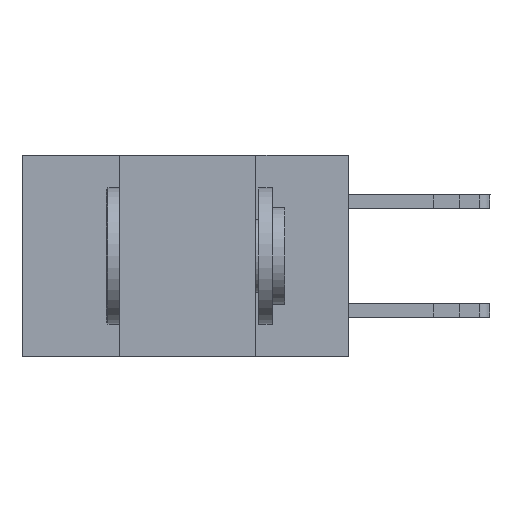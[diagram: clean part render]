
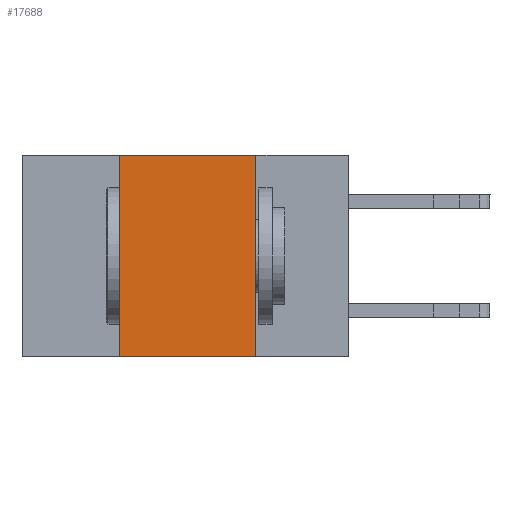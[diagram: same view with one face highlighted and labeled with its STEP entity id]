
A CAD part, left-side view. The second image highlights one B-rep face of the part: STEP entity #17688.
In plain terms, the highlighted planar face has unit normal (-1, 0, 0).
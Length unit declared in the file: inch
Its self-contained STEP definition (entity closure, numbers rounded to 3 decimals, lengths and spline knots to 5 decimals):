
#180 = DIRECTION ( 'NONE',  ( 1., 0., 0. ) ) ;
#474 = PLANE ( 'NONE',  #1665 ) ;
#1665 = AXIS2_PLACEMENT_3D ( 'NONE', #10974, #180, #7959 ) ;
#2076 = LINE ( 'NONE', #11078, #6819 ) ;
#2265 = EDGE_CURVE ( 'NONE', #10407, #18013, #8337, .T. ) ;
#2342 = CARTESIAN_POINT ( 'NONE',  ( 0., 0.17, 0. ) ) ;
#2468 = ORIENTED_EDGE ( 'NONE', *, *, #2265, .F. ) ;
#2672 = VECTOR ( 'NONE', #2863, 39.37008 ) ;
#2704 = CARTESIAN_POINT ( 'NONE',  ( 0., 0.6, -0.37 ) ) ;
#2863 = DIRECTION ( 'NONE',  ( 0., 0., 1. ) ) ;
#3048 = CARTESIAN_POINT ( 'NONE',  ( 0., 0.42, -0.37 ) ) ;
#3486 = DIRECTION ( 'NONE',  ( 0., -1., 0. ) ) ;
#4300 = ORIENTED_EDGE ( 'NONE', *, *, #19030, .F. ) ;
#5285 = CARTESIAN_POINT ( 'NONE',  ( 0., 0.17, 0. ) ) ;
#5636 = ORIENTED_EDGE ( 'NONE', *, *, #14462, .T. ) ;
#5957 = CARTESIAN_POINT ( 'NONE',  ( 0., 0.17, -0.37 ) ) ;
#6549 = DIRECTION ( 'NONE',  ( 0., 0., -1. ) ) ;
#6819 = VECTOR ( 'NONE', #3486, 39.37008 ) ;
#7959 = DIRECTION ( 'NONE',  ( 0., 0., -1. ) ) ;
#8313 = VECTOR ( 'NONE', #14998, 39.37008 ) ;
#8337 = LINE ( 'NONE', #2342, #15182 ) ;
#8905 = LINE ( 'NONE', #2704, #8313 ) ;
#9889 = EDGE_LOOP ( 'NONE', ( #2468, #4300, #11317, #5636 ) ) ;
#10407 = VERTEX_POINT ( 'NONE', #5285 ) ;
#10762 = LINE ( 'NONE', #15064, #2672 ) ;
#10974 = CARTESIAN_POINT ( 'NONE',  ( 0., 0.6, 0. ) ) ;
#11078 = CARTESIAN_POINT ( 'NONE',  ( 0., 0.6, 0. ) ) ;
#11168 = FACE_OUTER_BOUND ( 'NONE', #9889, .T. ) ;
#11317 = ORIENTED_EDGE ( 'NONE', *, *, #19286, .F. ) ;
#11823 = VERTEX_POINT ( 'NONE', #18587 ) ;
#14462 = EDGE_CURVE ( 'NONE', #15460, #18013, #8905, .T. ) ;
#14998 = DIRECTION ( 'NONE',  ( 0., -1., 0. ) ) ;
#15064 = CARTESIAN_POINT ( 'NONE',  ( 0., 0.42, 0. ) ) ;
#15182 = VECTOR ( 'NONE', #6549, 39.37008 ) ;
#15460 = VERTEX_POINT ( 'NONE', #3048 ) ;
#17688 = ADVANCED_FACE ( 'NONE', ( #11168 ), #474, .F. ) ;
#18013 = VERTEX_POINT ( 'NONE', #5957 ) ;
#18587 = CARTESIAN_POINT ( 'NONE',  ( 0., 0.42, 0. ) ) ;
#19030 = EDGE_CURVE ( 'NONE', #11823, #10407, #2076, .T. ) ;
#19286 = EDGE_CURVE ( 'NONE', #15460, #11823, #10762, .T. ) ;
